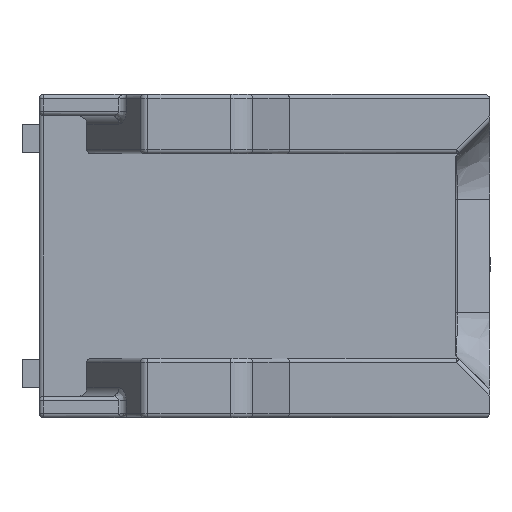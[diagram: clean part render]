
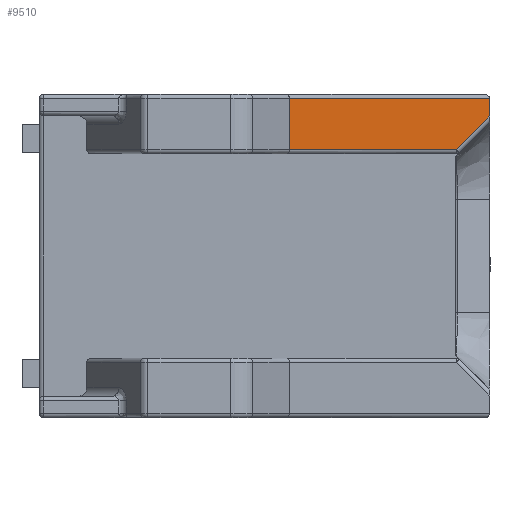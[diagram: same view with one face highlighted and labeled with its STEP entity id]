
A CAD part, left-side view. The second image highlights one B-rep face of the part: STEP entity #9510.
In plain terms, the highlighted planar face has unit normal (-1, 0, 0).
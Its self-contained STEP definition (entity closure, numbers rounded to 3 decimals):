
#372 = CARTESIAN_POINT ( 'NONE',  ( -84.9, -37.701, 19.5 ) ) ;
#935 = LINE ( 'NONE', #6570, #5944 ) ;
#1567 = LINE ( 'NONE', #13639, #16281 ) ;
#1929 = EDGE_CURVE ( 'NONE', #6951, #9037, #935, .T. ) ;
#2975 = DIRECTION ( 'NONE',  ( 0., 0., 1. ) ) ;
#3195 = LINE ( 'NONE', #4919, #12090 ) ;
#3203 = VECTOR ( 'NONE', #5695, 1000. ) ;
#3497 = FACE_OUTER_BOUND ( 'NONE', #7718, .T. ) ;
#3687 = CARTESIAN_POINT ( 'NONE',  ( -84.9, -61.29, 19.5 ) ) ;
#4044 = ORIENTED_EDGE ( 'NONE', *, *, #6415, .F. ) ;
#4532 = ORIENTED_EDGE ( 'NONE', *, *, #19157, .F. ) ;
#4919 = CARTESIAN_POINT ( 'NONE',  ( -84.9, -38.892, 13.5 ) ) ;
#5695 = DIRECTION ( 'NONE',  ( 0., -1., 0. ) ) ;
#5944 = VECTOR ( 'NONE', #17236, 1000. ) ;
#6352 = ORIENTED_EDGE ( 'NONE', *, *, #1929, .F. ) ;
#6415 = EDGE_CURVE ( 'NONE', #9037, #14378, #3195, .T. ) ;
#6570 = CARTESIAN_POINT ( 'NONE',  ( -84.9, -55.554, 11.721 ) ) ;
#6951 = VERTEX_POINT ( 'NONE', #8048 ) ;
#7155 = VERTEX_POINT ( 'NONE', #3687 ) ;
#7610 = LINE ( 'NONE', #14544, #3203 ) ;
#7718 = EDGE_LOOP ( 'NONE', ( #6352, #10896, #4532, #12490, #4044 ) ) ;
#8048 = CARTESIAN_POINT ( 'NONE',  ( -84.9, -61.29, 17.457 ) ) ;
#9037 = VERTEX_POINT ( 'NONE', #10531 ) ;
#9271 = EDGE_CURVE ( 'NONE', #6951, #7155, #1567, .T. ) ;
#9441 = DIRECTION ( 'NONE',  ( -1., 0., 0. ) ) ;
#9510 = ADVANCED_FACE ( 'NONE', ( #3497 ), #21343, .T. ) ;
#10438 = CARTESIAN_POINT ( 'NONE',  ( -84.9, -37.701, 13.5 ) ) ;
#10531 = CARTESIAN_POINT ( 'NONE',  ( -84.9, -57.333, 13.5 ) ) ;
#10896 = ORIENTED_EDGE ( 'NONE', *, *, #9271, .T. ) ;
#10944 = DIRECTION ( 'NONE',  ( 0., 0., -1. ) ) ;
#11268 = CARTESIAN_POINT ( 'NONE',  ( -84.9, -43.244, 17.266 ) ) ;
#11731 = EDGE_CURVE ( 'NONE', #17868, #14378, #15774, .T. ) ;
#12090 = VECTOR ( 'NONE', #19131, 1000. ) ;
#12490 = ORIENTED_EDGE ( 'NONE', *, *, #11731, .T. ) ;
#12596 = CARTESIAN_POINT ( 'NONE',  ( -84.9, -37.701, 15.533 ) ) ;
#13639 = CARTESIAN_POINT ( 'NONE',  ( -84.9, -61.29, 17.303 ) ) ;
#14378 = VERTEX_POINT ( 'NONE', #10438 ) ;
#14544 = CARTESIAN_POINT ( 'NONE',  ( -84.9, -38.892, 19.5 ) ) ;
#15427 = AXIS2_PLACEMENT_3D ( 'NONE', #11268, #9441, #19971 ) ;
#15774 = LINE ( 'NONE', #12596, #16325 ) ;
#16281 = VECTOR ( 'NONE', #2975, 1000. ) ;
#16325 = VECTOR ( 'NONE', #10944, 1000. ) ;
#17236 = DIRECTION ( 'NONE',  ( 0., 0.707, -0.707 ) ) ;
#17868 = VERTEX_POINT ( 'NONE', #372 ) ;
#19131 = DIRECTION ( 'NONE',  ( 0., 1., 0. ) ) ;
#19157 = EDGE_CURVE ( 'NONE', #17868, #7155, #7610, .T. ) ;
#19971 = DIRECTION ( 'NONE',  ( 0., 1., 0. ) ) ;
#21343 = PLANE ( 'NONE',  #15427 ) ;
